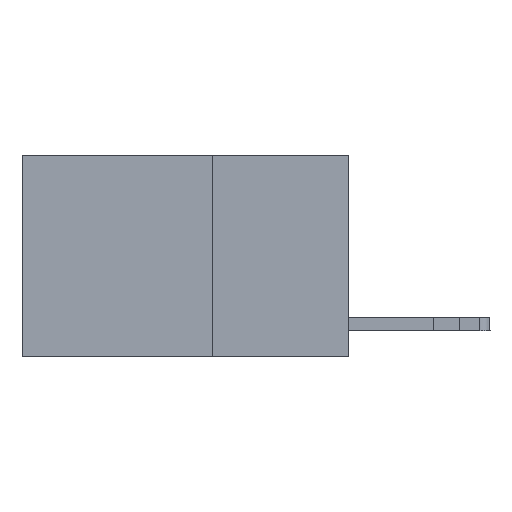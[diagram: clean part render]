
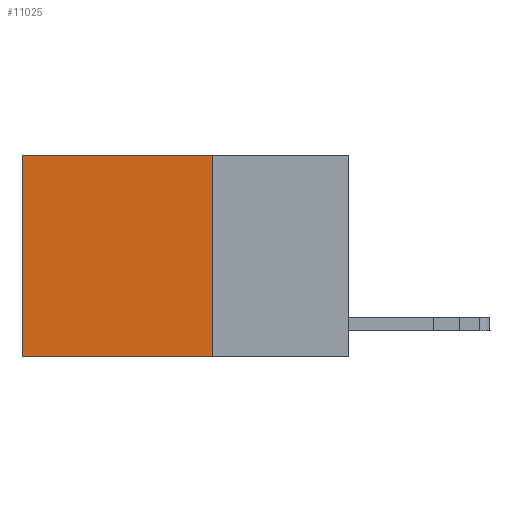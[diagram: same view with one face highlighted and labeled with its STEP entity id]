
A CAD part, left-side view. The second image highlights one B-rep face of the part: STEP entity #11025.
In plain terms, the highlighted planar face has unit normal (-1, 0, 0).
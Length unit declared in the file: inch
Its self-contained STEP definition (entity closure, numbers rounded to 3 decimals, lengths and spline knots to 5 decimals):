
#57 = DIRECTION ( 'NONE',  ( 0., 1., 0. ) ) ;
#379 = ORIENTED_EDGE ( 'NONE', *, *, #22932, .F. ) ;
#1543 = AXIS2_PLACEMENT_3D ( 'NONE', #5915, #11381, #4302 ) ;
#2345 = VECTOR ( 'NONE', #5462, 39.37008 ) ;
#4302 = DIRECTION ( 'NONE',  ( 0., 0., -1. ) ) ;
#4304 = VERTEX_POINT ( 'NONE', #12763 ) ;
#5289 = EDGE_CURVE ( 'NONE', #4304, #13392, #11214, .T. ) ;
#5462 = DIRECTION ( 'NONE',  ( 0., 1., 0. ) ) ;
#5668 = EDGE_LOOP ( 'NONE', ( #16557, #17586, #379, #11768 ) ) ;
#5915 = CARTESIAN_POINT ( 'NONE',  ( 0.2625, 0.25, 0. ) ) ;
#7999 = VERTEX_POINT ( 'NONE', #14805 ) ;
#8135 = VECTOR ( 'NONE', #16719, 39.37008 ) ;
#8542 = CARTESIAN_POINT ( 'NONE',  ( 0.2625, 0.25, 0. ) ) ;
#9592 = CARTESIAN_POINT ( 'NONE',  ( 0.2625, 0.6, 0. ) ) ;
#10730 = CARTESIAN_POINT ( 'NONE',  ( 0.2625, 0.6, -0.37 ) ) ;
#11025 = ADVANCED_FACE ( 'NONE', ( #11615 ), #16535, .F. ) ;
#11214 = LINE ( 'NONE', #9592, #8135 ) ;
#11381 = DIRECTION ( 'NONE',  ( 1., 0., 0. ) ) ;
#11615 = FACE_OUTER_BOUND ( 'NONE', #5668, .T. ) ;
#11768 = ORIENTED_EDGE ( 'NONE', *, *, #19931, .T. ) ;
#12239 = DIRECTION ( 'NONE',  ( 0., 0., -1. ) ) ;
#12354 = CARTESIAN_POINT ( 'NONE',  ( 0.2625, 0.25, -0.37 ) ) ;
#12763 = CARTESIAN_POINT ( 'NONE',  ( 0.2625, 0.6, 0. ) ) ;
#12859 = VERTEX_POINT ( 'NONE', #15310 ) ;
#13362 = EDGE_CURVE ( 'NONE', #7999, #13392, #21157, .T. ) ;
#13392 = VERTEX_POINT ( 'NONE', #10730 ) ;
#14085 = LINE ( 'NONE', #17635, #2345 ) ;
#14805 = CARTESIAN_POINT ( 'NONE',  ( 0.2625, 0.25, -0.37 ) ) ;
#15310 = CARTESIAN_POINT ( 'NONE',  ( 0.2625, 0.25, 0. ) ) ;
#16535 = PLANE ( 'NONE',  #1543 ) ;
#16557 = ORIENTED_EDGE ( 'NONE', *, *, #5289, .T. ) ;
#16719 = DIRECTION ( 'NONE',  ( 0., 0., -1. ) ) ;
#17467 = VECTOR ( 'NONE', #57, 39.37008 ) ;
#17586 = ORIENTED_EDGE ( 'NONE', *, *, #13362, .F. ) ;
#17635 = CARTESIAN_POINT ( 'NONE',  ( 0.2625, 0.25, 0. ) ) ;
#19075 = LINE ( 'NONE', #8542, #20407 ) ;
#19931 = EDGE_CURVE ( 'NONE', #12859, #4304, #14085, .T. ) ;
#20407 = VECTOR ( 'NONE', #12239, 39.37008 ) ;
#21157 = LINE ( 'NONE', #12354, #17467 ) ;
#22932 = EDGE_CURVE ( 'NONE', #12859, #7999, #19075, .T. ) ;
